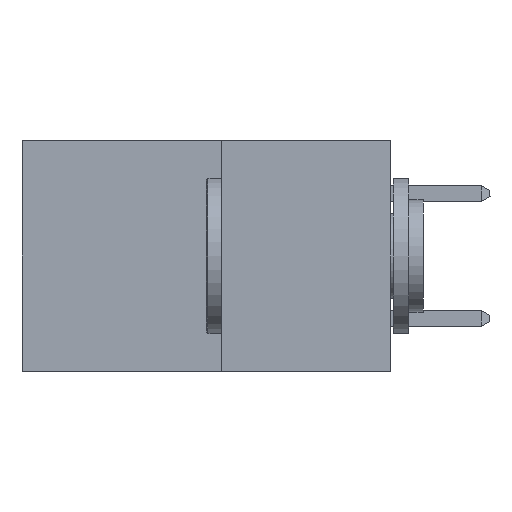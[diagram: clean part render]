
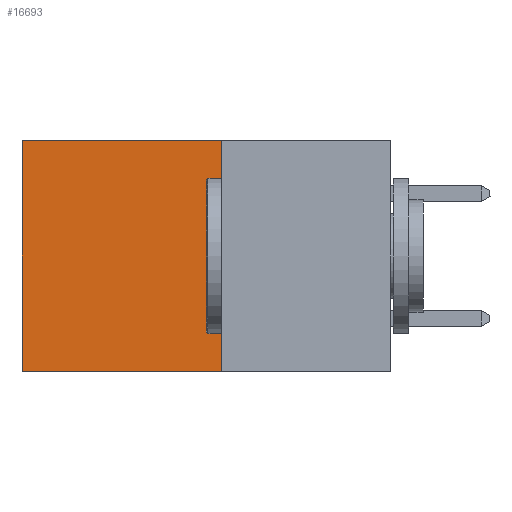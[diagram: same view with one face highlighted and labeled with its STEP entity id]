
A CAD part, left-side view. The second image highlights one B-rep face of the part: STEP entity #16693.
In plain terms, the highlighted planar face has unit normal (-1, 0, 0).
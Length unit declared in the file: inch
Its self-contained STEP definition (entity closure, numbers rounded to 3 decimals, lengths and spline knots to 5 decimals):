
#267 = EDGE_LOOP ( 'NONE', ( #1555, #14685, #15120, #1986 ) ) ;
#269 = VECTOR ( 'NONE', #6437, 39.37008 ) ;
#461 = DIRECTION ( 'NONE',  ( 0., 1., 0. ) ) ;
#732 = CARTESIAN_POINT ( 'NONE',  ( 0.277, 0.59, -0.37 ) ) ;
#1555 = ORIENTED_EDGE ( 'NONE', *, *, #7110, .T. ) ;
#1986 = ORIENTED_EDGE ( 'NONE', *, *, #15011, .T. ) ;
#2107 = PLANE ( 'NONE',  #5153 ) ;
#2397 = LINE ( 'NONE', #10028, #12793 ) ;
#2471 = EDGE_CURVE ( 'NONE', #3099, #5665, #11524, .T. ) ;
#2611 = CARTESIAN_POINT ( 'NONE',  ( 0.277, 0.27, 0. ) ) ;
#3099 = VERTEX_POINT ( 'NONE', #2611 ) ;
#3524 = DIRECTION ( 'NONE',  ( 1., 0., 0. ) ) ;
#3889 = VECTOR ( 'NONE', #4357, 39.37008 ) ;
#4357 = DIRECTION ( 'NONE',  ( 0., 1., 0. ) ) ;
#4691 = CARTESIAN_POINT ( 'NONE',  ( 0.277, 0.27, -0.37 ) ) ;
#5153 = AXIS2_PLACEMENT_3D ( 'NONE', #11648, #3524, #12977 ) ;
#5665 = VERTEX_POINT ( 'NONE', #4691 ) ;
#6437 = DIRECTION ( 'NONE',  ( 0., 0., -1. ) ) ;
#6533 = CARTESIAN_POINT ( 'NONE',  ( 0.277, 0.59, -0.37 ) ) ;
#7110 = EDGE_CURVE ( 'NONE', #9336, #13036, #11177, .T. ) ;
#8310 = CARTESIAN_POINT ( 'NONE',  ( 0.277, 0.59, 0. ) ) ;
#9336 = VERTEX_POINT ( 'NONE', #8310 ) ;
#10028 = CARTESIAN_POINT ( 'NONE',  ( 0.277, 0.27, -0.37 ) ) ;
#11114 = LINE ( 'NONE', #16257, #3889 ) ;
#11177 = LINE ( 'NONE', #6533, #269 ) ;
#11257 = FACE_OUTER_BOUND ( 'NONE', #267, .T. ) ;
#11450 = DIRECTION ( 'NONE',  ( 0., 0., -1. ) ) ;
#11524 = LINE ( 'NONE', #15133, #14959 ) ;
#11648 = CARTESIAN_POINT ( 'NONE',  ( 0.277, 0.27, -0.37 ) ) ;
#12793 = VECTOR ( 'NONE', #461, 39.37008 ) ;
#12977 = DIRECTION ( 'NONE',  ( 0., 0., -1. ) ) ;
#13036 = VERTEX_POINT ( 'NONE', #732 ) ;
#13504 = EDGE_CURVE ( 'NONE', #5665, #13036, #2397, .T. ) ;
#14685 = ORIENTED_EDGE ( 'NONE', *, *, #13504, .F. ) ;
#14959 = VECTOR ( 'NONE', #11450, 39.37008 ) ;
#15011 = EDGE_CURVE ( 'NONE', #3099, #9336, #11114, .T. ) ;
#15120 = ORIENTED_EDGE ( 'NONE', *, *, #2471, .F. ) ;
#15133 = CARTESIAN_POINT ( 'NONE',  ( 0.277, 0.27, -0.37 ) ) ;
#16257 = CARTESIAN_POINT ( 'NONE',  ( 0.277, 0.27, 0. ) ) ;
#16693 = ADVANCED_FACE ( 'NONE', ( #11257 ), #2107, .F. ) ;
